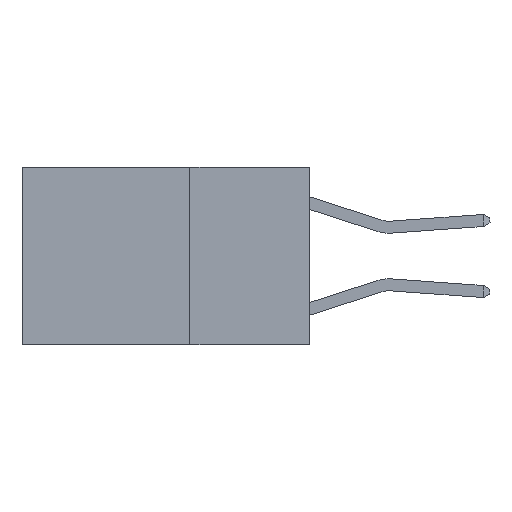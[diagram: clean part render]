
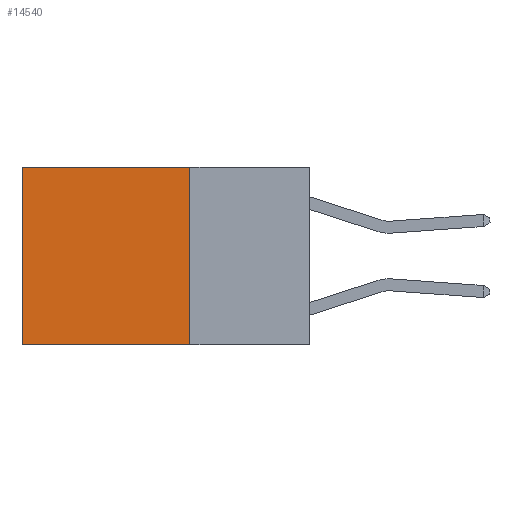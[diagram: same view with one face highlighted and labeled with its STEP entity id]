
A CAD part, left-side view. The second image highlights one B-rep face of the part: STEP entity #14540.
In plain terms, the highlighted planar face has unit normal (-1, 0, 0).
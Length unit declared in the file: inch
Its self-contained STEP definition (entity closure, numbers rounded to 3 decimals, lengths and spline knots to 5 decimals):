
#313 = LINE ( 'NONE', #5493, #11305 ) ;
#361 = EDGE_CURVE ( 'NONE', #9379, #21768, #6854, .T. ) ;
#1378 = CARTESIAN_POINT ( 'NONE',  ( 0.2625, 0.25, -0.37 ) ) ;
#1812 = LINE ( 'NONE', #9387, #17699 ) ;
#2116 = CARTESIAN_POINT ( 'NONE',  ( 0.2625, 0.25, 0. ) ) ;
#2571 = DIRECTION ( 'NONE',  ( 0., 1., 0. ) ) ;
#2743 = CARTESIAN_POINT ( 'NONE',  ( 0.2625, 0.25, 0. ) ) ;
#3128 = ORIENTED_EDGE ( 'NONE', *, *, #361, .T. ) ;
#3149 = CARTESIAN_POINT ( 'NONE',  ( 0.2625, 0.6, 0. ) ) ;
#3498 = CARTESIAN_POINT ( 'NONE',  ( 0.2625, 0.6, -0.37 ) ) ;
#4288 = DIRECTION ( 'NONE',  ( 0., 1., 0. ) ) ;
#4710 = VECTOR ( 'NONE', #19210, 39.37008 ) ;
#4888 = AXIS2_PLACEMENT_3D ( 'NONE', #15916, #19202, #8840 ) ;
#5272 = PLANE ( 'NONE',  #4888 ) ;
#5454 = EDGE_CURVE ( 'NONE', #21768, #12084, #313, .T. ) ;
#5493 = CARTESIAN_POINT ( 'NONE',  ( 0.2625, 0.6, 0. ) ) ;
#6854 = LINE ( 'NONE', #15976, #10867 ) ;
#7156 = FACE_OUTER_BOUND ( 'NONE', #21183, .T. ) ;
#8413 = EDGE_CURVE ( 'NONE', #9379, #17395, #16058, .T. ) ;
#8761 = DIRECTION ( 'NONE',  ( 0., 0., -1. ) ) ;
#8840 = DIRECTION ( 'NONE',  ( 0., 0., -1. ) ) ;
#9379 = VERTEX_POINT ( 'NONE', #2743 ) ;
#9387 = CARTESIAN_POINT ( 'NONE',  ( 0.2625, 0.25, -0.37 ) ) ;
#10867 = VECTOR ( 'NONE', #4288, 39.37008 ) ;
#11305 = VECTOR ( 'NONE', #8761, 39.37008 ) ;
#12023 = ORIENTED_EDGE ( 'NONE', *, *, #14212, .F. ) ;
#12084 = VERTEX_POINT ( 'NONE', #3498 ) ;
#14212 = EDGE_CURVE ( 'NONE', #17395, #12084, #1812, .T. ) ;
#14540 = ADVANCED_FACE ( 'NONE', ( #7156 ), #5272, .F. ) ;
#15916 = CARTESIAN_POINT ( 'NONE',  ( 0.2625, 0.25, 0. ) ) ;
#15976 = CARTESIAN_POINT ( 'NONE',  ( 0.2625, 0.25, 0. ) ) ;
#16058 = LINE ( 'NONE', #2116, #4710 ) ;
#17395 = VERTEX_POINT ( 'NONE', #1378 ) ;
#17699 = VECTOR ( 'NONE', #2571, 39.37008 ) ;
#18780 = ORIENTED_EDGE ( 'NONE', *, *, #8413, .F. ) ;
#19202 = DIRECTION ( 'NONE',  ( 1., 0., 0. ) ) ;
#19210 = DIRECTION ( 'NONE',  ( 0., 0., -1. ) ) ;
#20549 = ORIENTED_EDGE ( 'NONE', *, *, #5454, .T. ) ;
#21183 = EDGE_LOOP ( 'NONE', ( #20549, #12023, #18780, #3128 ) ) ;
#21768 = VERTEX_POINT ( 'NONE', #3149 ) ;
